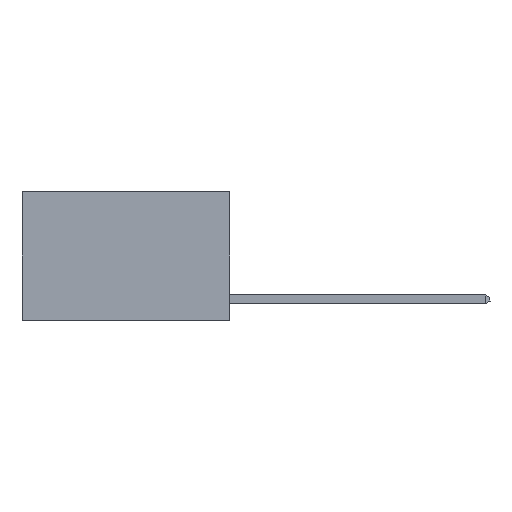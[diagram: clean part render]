
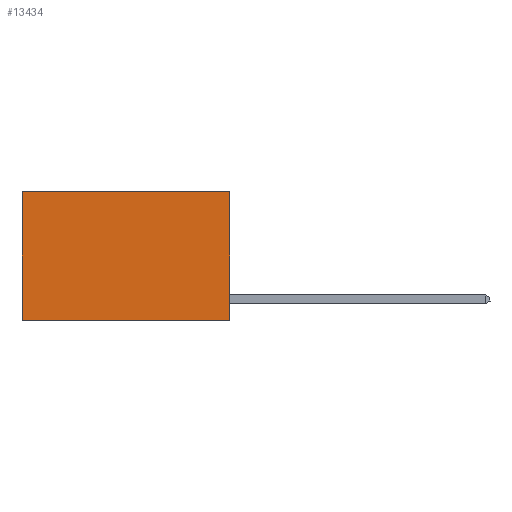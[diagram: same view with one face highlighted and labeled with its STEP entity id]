
A CAD part, left-side view. The second image highlights one B-rep face of the part: STEP entity #13434.
In plain terms, the highlighted planar face has unit normal (-1, 0, 0).
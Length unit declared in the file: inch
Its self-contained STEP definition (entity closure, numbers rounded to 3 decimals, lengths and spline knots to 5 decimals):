
#9 = CARTESIAN_POINT ( 'NONE',  ( 0.2625, 0., 0. ) ) ;
#143 = CARTESIAN_POINT ( 'NONE',  ( 0.2625, 0., 0. ) ) ;
#1702 = DIRECTION ( 'NONE',  ( 0., 0., -1. ) ) ;
#1869 = ORIENTED_EDGE ( 'NONE', *, *, #10251, .F. ) ;
#2028 = CARTESIAN_POINT ( 'NONE',  ( 0.2625, 0.6, -0.37 ) ) ;
#2305 = EDGE_CURVE ( 'NONE', #2644, #12500, #8086, .T. ) ;
#2644 = VERTEX_POINT ( 'NONE', #143 ) ;
#3130 = CARTESIAN_POINT ( 'NONE',  ( 0.2625, 0.6, 0. ) ) ;
#4372 = VECTOR ( 'NONE', #8667, 39.37008 ) ;
#5178 = CARTESIAN_POINT ( 'NONE',  ( 0.2625, 0., 0. ) ) ;
#5223 = EDGE_CURVE ( 'NONE', #17626, #8038, #6969, .T. ) ;
#5585 = EDGE_LOOP ( 'NONE', ( #7958, #1869, #10074, #16014 ) ) ;
#6501 = VECTOR ( 'NONE', #12850, 39.37008 ) ;
#6666 = DIRECTION ( 'NONE',  ( 0., 0., -1. ) ) ;
#6715 = VECTOR ( 'NONE', #8233, 39.37008 ) ;
#6969 = LINE ( 'NONE', #20221, #10932 ) ;
#7249 = LINE ( 'NONE', #16687, #6715 ) ;
#7776 = CARTESIAN_POINT ( 'NONE',  ( 0.2625, 0., 0. ) ) ;
#7958 = ORIENTED_EDGE ( 'NONE', *, *, #5223, .T. ) ;
#8038 = VERTEX_POINT ( 'NONE', #2028 ) ;
#8086 = LINE ( 'NONE', #7776, #6501 ) ;
#8233 = DIRECTION ( 'NONE',  ( 0., 1., 0. ) ) ;
#8460 = FACE_OUTER_BOUND ( 'NONE', #5585, .T. ) ;
#8667 = DIRECTION ( 'NONE',  ( 0., 1., 0. ) ) ;
#10074 = ORIENTED_EDGE ( 'NONE', *, *, #2305, .F. ) ;
#10251 = EDGE_CURVE ( 'NONE', #12500, #8038, #7249, .T. ) ;
#10932 = VECTOR ( 'NONE', #6666, 39.37008 ) ;
#11820 = DIRECTION ( 'NONE',  ( 1., 0., 0. ) ) ;
#12500 = VERTEX_POINT ( 'NONE', #20982 ) ;
#12850 = DIRECTION ( 'NONE',  ( 0., 0., -1. ) ) ;
#13434 = ADVANCED_FACE ( 'NONE', ( #8460 ), #16891, .F. ) ;
#15244 = EDGE_CURVE ( 'NONE', #2644, #17626, #17925, .T. ) ;
#16014 = ORIENTED_EDGE ( 'NONE', *, *, #15244, .T. ) ;
#16687 = CARTESIAN_POINT ( 'NONE',  ( 0.2625, 0., -0.37 ) ) ;
#16891 = PLANE ( 'NONE',  #17703 ) ;
#17626 = VERTEX_POINT ( 'NONE', #3130 ) ;
#17703 = AXIS2_PLACEMENT_3D ( 'NONE', #9, #11820, #1702 ) ;
#17925 = LINE ( 'NONE', #5178, #4372 ) ;
#20221 = CARTESIAN_POINT ( 'NONE',  ( 0.2625, 0.6, 0. ) ) ;
#20982 = CARTESIAN_POINT ( 'NONE',  ( 0.2625, 0., -0.37 ) ) ;
